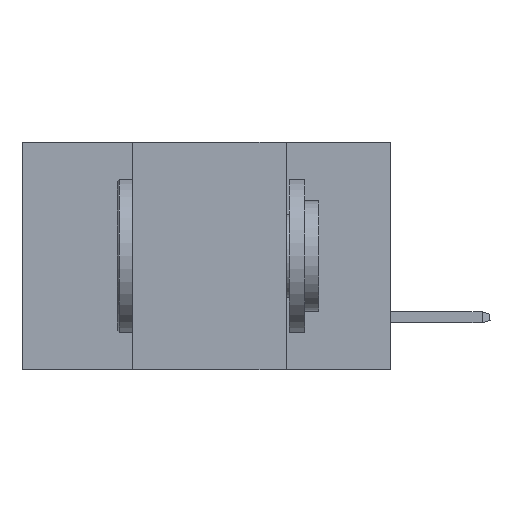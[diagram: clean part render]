
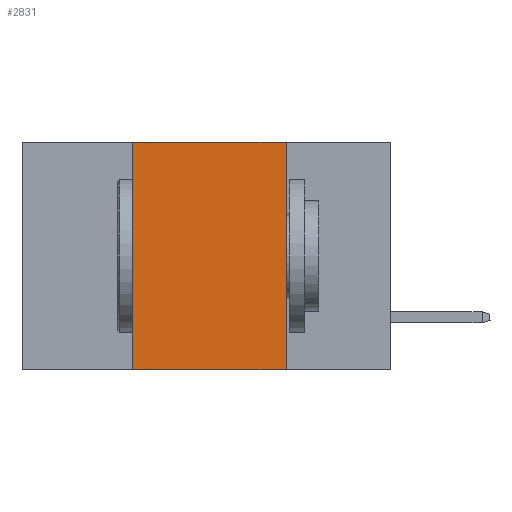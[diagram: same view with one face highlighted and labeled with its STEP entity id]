
A CAD part, left-side view. The second image highlights one B-rep face of the part: STEP entity #2831.
In plain terms, the highlighted planar face has unit normal (-1, 0, 0).
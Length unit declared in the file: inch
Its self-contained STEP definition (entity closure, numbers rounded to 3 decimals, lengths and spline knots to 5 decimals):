
#571 = VERTEX_POINT ( 'NONE', #9325 ) ;
#672 = DIRECTION ( 'NONE',  ( 0., 0., -1. ) ) ;
#975 = DIRECTION ( 'NONE',  ( 0., 0., -1. ) ) ;
#2038 = CARTESIAN_POINT ( 'NONE',  ( 0., 0.42, 0. ) ) ;
#2275 = ORIENTED_EDGE ( 'NONE', *, *, #12238, .F. ) ;
#2618 = VERTEX_POINT ( 'NONE', #13846 ) ;
#2831 = ADVANCED_FACE ( 'NONE', ( #14187 ), #4729, .F. ) ;
#3352 = VERTEX_POINT ( 'NONE', #3602 ) ;
#3602 = CARTESIAN_POINT ( 'NONE',  ( 0., 0.17, -0.37 ) ) ;
#4035 = VECTOR ( 'NONE', #10095, 39.37008 ) ;
#4343 = VECTOR ( 'NONE', #20850, 39.37008 ) ;
#4729 = PLANE ( 'NONE',  #16980 ) ;
#5799 = EDGE_LOOP ( 'NONE', ( #2275, #23798, #20872, #7938 ) ) ;
#7317 = DIRECTION ( 'NONE',  ( 0., -1., 0. ) ) ;
#7938 = ORIENTED_EDGE ( 'NONE', *, *, #21704, .T. ) ;
#9325 = CARTESIAN_POINT ( 'NONE',  ( 0., 0.17, 0. ) ) ;
#10095 = DIRECTION ( 'NONE',  ( 0., -1., 0. ) ) ;
#11267 = LINE ( 'NONE', #13950, #23076 ) ;
#12238 = EDGE_CURVE ( 'NONE', #571, #3352, #11267, .T. ) ;
#13061 = CARTESIAN_POINT ( 'NONE',  ( 0., 0.42, -0.37 ) ) ;
#13846 = CARTESIAN_POINT ( 'NONE',  ( 0., 0.42, 0. ) ) ;
#13950 = CARTESIAN_POINT ( 'NONE',  ( 0., 0.17, 0. ) ) ;
#14086 = LINE ( 'NONE', #21445, #4035 ) ;
#14187 = FACE_OUTER_BOUND ( 'NONE', #5799, .T. ) ;
#15102 = EDGE_CURVE ( 'NONE', #15705, #2618, #21791, .T. ) ;
#15370 = EDGE_CURVE ( 'NONE', #2618, #571, #14086, .T. ) ;
#15705 = VERTEX_POINT ( 'NONE', #13061 ) ;
#16150 = CARTESIAN_POINT ( 'NONE',  ( 0., 0.6, 0. ) ) ;
#16980 = AXIS2_PLACEMENT_3D ( 'NONE', #16150, #19977, #975 ) ;
#18133 = VECTOR ( 'NONE', #7317, 39.37008 ) ;
#18750 = LINE ( 'NONE', #21687, #18133 ) ;
#19977 = DIRECTION ( 'NONE',  ( 1., 0., 0. ) ) ;
#20850 = DIRECTION ( 'NONE',  ( 0., 0., 1. ) ) ;
#20872 = ORIENTED_EDGE ( 'NONE', *, *, #15102, .F. ) ;
#21445 = CARTESIAN_POINT ( 'NONE',  ( 0., 0.6, 0. ) ) ;
#21687 = CARTESIAN_POINT ( 'NONE',  ( 0., 0.6, -0.37 ) ) ;
#21704 = EDGE_CURVE ( 'NONE', #15705, #3352, #18750, .T. ) ;
#21791 = LINE ( 'NONE', #2038, #4343 ) ;
#23076 = VECTOR ( 'NONE', #672, 39.37008 ) ;
#23798 = ORIENTED_EDGE ( 'NONE', *, *, #15370, .F. ) ;
